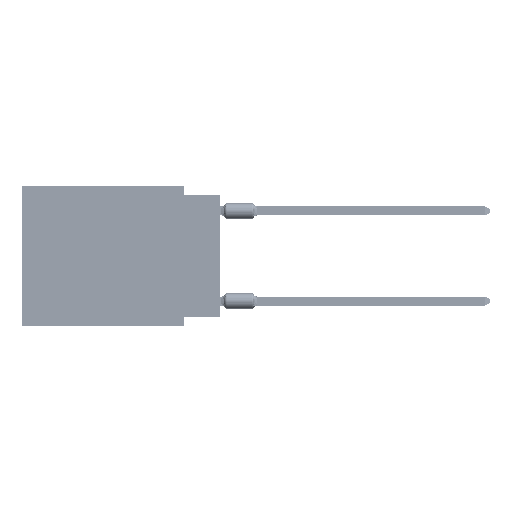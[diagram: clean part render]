
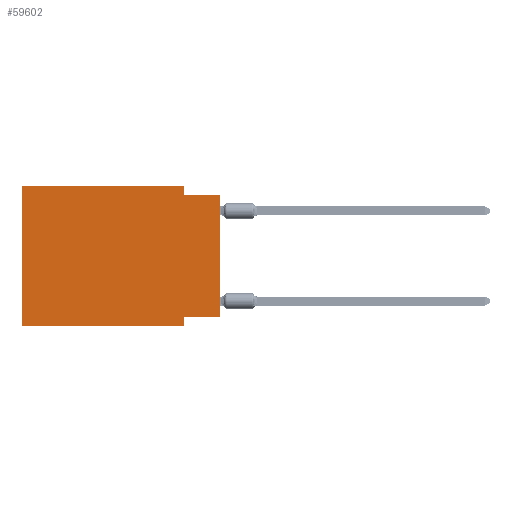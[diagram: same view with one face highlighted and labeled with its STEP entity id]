
A CAD part, left-side view. The second image highlights one B-rep face of the part: STEP entity #59602.
In plain terms, the highlighted planar face has unit normal (-1, 0, 0).
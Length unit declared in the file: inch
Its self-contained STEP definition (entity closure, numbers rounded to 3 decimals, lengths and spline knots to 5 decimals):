
#1997 = DIRECTION ( 'NONE',  ( 0., 0., 1. ) ) ;
#2314 = EDGE_LOOP ( 'NONE', ( #15972, #20544, #45214, #46843, #36678, #70693, #15360, #65191 ) ) ;
#3304 = LINE ( 'NONE', #52346, #55109 ) ;
#4931 = LINE ( 'NONE', #58018, #68968 ) ;
#6400 = LINE ( 'NONE', #43473, #38000 ) ;
#6482 = EDGE_CURVE ( 'NONE', #58839, #11465, #59256, .T. ) ;
#7321 = CARTESIAN_POINT ( 'NONE',  ( 0., 0.1, -0.365 ) ) ;
#8888 = CARTESIAN_POINT ( 'NONE',  ( 0., 0.1, -0.39 ) ) ;
#11465 = VERTEX_POINT ( 'NONE', #41471 ) ;
#12098 = EDGE_CURVE ( 'NONE', #59007, #23419, #18903, .T. ) ;
#12835 = DIRECTION ( 'NONE',  ( 1., 0., 0. ) ) ;
#13430 = DIRECTION ( 'NONE',  ( 0., -1., 0. ) ) ;
#14208 = LINE ( 'NONE', #68079, #40645 ) ;
#15360 = ORIENTED_EDGE ( 'NONE', *, *, #16800, .F. ) ;
#15423 = VERTEX_POINT ( 'NONE', #7321 ) ;
#15972 = ORIENTED_EDGE ( 'NONE', *, *, #67167, .T. ) ;
#16047 = CARTESIAN_POINT ( 'NONE',  ( 0., 0., -0.365 ) ) ;
#16344 = DIRECTION ( 'NONE',  ( 0., -1., 0. ) ) ;
#16800 = EDGE_CURVE ( 'NONE', #15423, #19041, #3304, .T. ) ;
#18903 = LINE ( 'NONE', #44023, #72448 ) ;
#19041 = VERTEX_POINT ( 'NONE', #8888 ) ;
#20544 = ORIENTED_EDGE ( 'NONE', *, *, #32125, .F. ) ;
#21552 = EDGE_CURVE ( 'NONE', #59007, #19041, #14208, .T. ) ;
#23419 = VERTEX_POINT ( 'NONE', #41731 ) ;
#26060 = VECTOR ( 'NONE', #16344, 39.37008 ) ;
#27144 = DIRECTION ( 'NONE',  ( 0., -1., 0. ) ) ;
#28332 = CARTESIAN_POINT ( 'NONE',  ( 0., 0.55, 0. ) ) ;
#28949 = VERTEX_POINT ( 'NONE', #16047 ) ;
#31438 = CARTESIAN_POINT ( 'NONE',  ( 0., 0.1, 0. ) ) ;
#32125 = EDGE_CURVE ( 'NONE', #11465, #56157, #47032, .T. ) ;
#34388 = DIRECTION ( 'NONE',  ( 0., 0., -1. ) ) ;
#35940 = VECTOR ( 'NONE', #47273, 39.37008 ) ;
#36678 = ORIENTED_EDGE ( 'NONE', *, *, #12098, .F. ) ;
#36743 = PLANE ( 'NONE',  #73640 ) ;
#38000 = VECTOR ( 'NONE', #1997, 39.37008 ) ;
#39580 = EDGE_CURVE ( 'NONE', #23419, #58839, #51509, .T. ) ;
#40645 = VECTOR ( 'NONE', #13430, 39.37008 ) ;
#40905 = EDGE_CURVE ( 'NONE', #28949, #15423, #4931, .T. ) ;
#41471 = CARTESIAN_POINT ( 'NONE',  ( 0., 0.1, -0.025 ) ) ;
#41731 = CARTESIAN_POINT ( 'NONE',  ( 0., 0.55, 0. ) ) ;
#43473 = CARTESIAN_POINT ( 'NONE',  ( 0., 0., 0. ) ) ;
#44023 = CARTESIAN_POINT ( 'NONE',  ( 0., 0.55, 0. ) ) ;
#45214 = ORIENTED_EDGE ( 'NONE', *, *, #6482, .F. ) ;
#45377 = CARTESIAN_POINT ( 'NONE',  ( 0., 0.55, -0.39 ) ) ;
#46843 = ORIENTED_EDGE ( 'NONE', *, *, #39580, .F. ) ;
#47032 = LINE ( 'NONE', #71009, #26060 ) ;
#47273 = DIRECTION ( 'NONE',  ( 0., 0., -1. ) ) ;
#49838 = CARTESIAN_POINT ( 'NONE',  ( 0., 0., -0.025 ) ) ;
#51509 = LINE ( 'NONE', #28332, #54789 ) ;
#52346 = CARTESIAN_POINT ( 'NONE',  ( 0., 0.1, -0.39 ) ) ;
#53580 = DIRECTION ( 'NONE',  ( 0., 1., 0. ) ) ;
#54789 = VECTOR ( 'NONE', #27144, 39.37008 ) ;
#55109 = VECTOR ( 'NONE', #34388, 39.37008 ) ;
#55108 = CARTESIAN_POINT ( 'NONE',  ( 0., 0.55, 0. ) ) ;
#56157 = VERTEX_POINT ( 'NONE', #49838 ) ;
#58018 = CARTESIAN_POINT ( 'NONE',  ( 0., 0., -0.365 ) ) ;
#58839 = VERTEX_POINT ( 'NONE', #31438 ) ;
#59007 = VERTEX_POINT ( 'NONE', #45377 ) ;
#59256 = LINE ( 'NONE', #76427, #35940 ) ;
#59602 = ADVANCED_FACE ( 'NONE', ( #68662 ), #36743, .F. ) ;
#65191 = ORIENTED_EDGE ( 'NONE', *, *, #40905, .F. ) ;
#67167 = EDGE_CURVE ( 'NONE', #28949, #56157, #6400, .T. ) ;
#67584 = DIRECTION ( 'NONE',  ( 0., 0., 1. ) ) ;
#68079 = CARTESIAN_POINT ( 'NONE',  ( 0., 0.55, -0.39 ) ) ;
#68270 = DIRECTION ( 'NONE',  ( 0., 0., -1. ) ) ;
#68662 = FACE_OUTER_BOUND ( 'NONE', #2314, .T. ) ;
#68968 = VECTOR ( 'NONE', #53580, 39.37008 ) ;
#70693 = ORIENTED_EDGE ( 'NONE', *, *, #21552, .T. ) ;
#71009 = CARTESIAN_POINT ( 'NONE',  ( 0., 0., -0.025 ) ) ;
#72448 = VECTOR ( 'NONE', #67584, 39.37008 ) ;
#73640 = AXIS2_PLACEMENT_3D ( 'NONE', #55108, #12835, #68270 ) ;
#76427 = CARTESIAN_POINT ( 'NONE',  ( 0., 0.1, 0. ) ) ;
